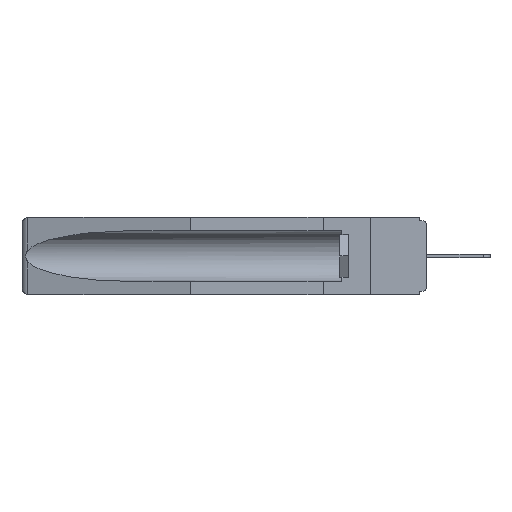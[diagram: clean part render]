
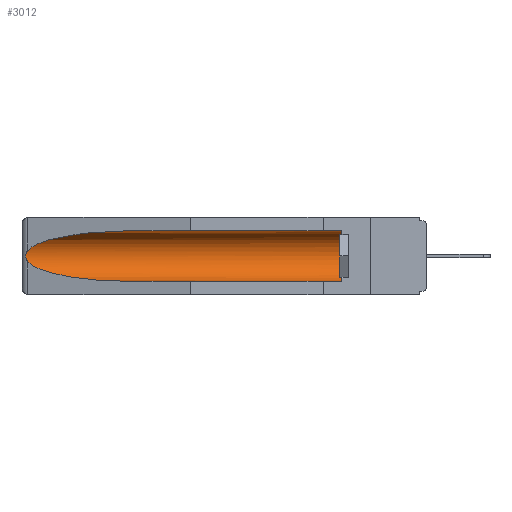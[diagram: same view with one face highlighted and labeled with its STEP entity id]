
A CAD part, left-side view. The second image highlights one B-rep face of the part: STEP entity #3012.
In plain terms, the highlighted cylindrical face has radius 2.857 mm (diameter 5.715 mm), a partial arc.
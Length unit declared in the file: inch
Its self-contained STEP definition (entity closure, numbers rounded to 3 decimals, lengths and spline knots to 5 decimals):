
#176 = CARTESIAN_POINT ( 'NONE',  ( 0.155, -0.30754, -0.284 ) ) ;
#478 = CARTESIAN_POINT ( 'NONE',  ( 0.2673, 1.5327, -0.16383 ) ) ;
#628 = CARTESIAN_POINT ( 'NONE',  ( 0.26654, 1.53092, -0.15636 ) ) ;
#876 = FACE_OUTER_BOUND ( 'NONE', #15188, .T. ) ;
#1124 = VERTEX_POINT ( 'NONE', #7832 ) ;
#1272 = CARTESIAN_POINT ( 'NONE',  ( 0.155, -0.30754, -0.1715 ) ) ;
#1479 =( BOUNDED_CURVE ( )  B_SPLINE_CURVE ( 3, ( #5331, #14253, #7152, #3442 ),
 .UNSPECIFIED., .F., .T. ) 
 B_SPLINE_CURVE_WITH_KNOTS ( ( 4, 4 ),
 ( 4.71239, 6.08839 ),
 .UNSPECIFIED. ) 
 CURVE ( )  GEOMETRIC_REPRESENTATION_ITEM ( )  RATIONAL_B_SPLINE_CURVE ( ( 1., 0.848, 0.848, 1. ) ) 
 REPRESENTATION_ITEM ( '' )  );
#1482 = VECTOR ( 'NONE', #19465, 39.37008 ) ;
#2046 = AXIS2_PLACEMENT_3D ( 'NONE', #1272, #12177, #14144 ) ;
#2461 = CARTESIAN_POINT ( 'NONE',  ( 0.26597, 1.5296, -0.19026 ) ) ;
#2616 = CARTESIAN_POINT ( 'NONE',  ( 0.155, 0.126, -0.059 ) ) ;
#3012 = ADVANCED_FACE ( 'NONE', ( #876 ), #17522, .F. ) ;
#3419 = DIRECTION ( 'NONE',  ( 0., 1., 0. ) ) ;
#3442 = CARTESIAN_POINT ( 'NONE',  ( 0.26537, 1.52718, -0.14972 ) ) ;
#3687 = LINE ( 'NONE', #176, #17489 ) ;
#4626 = B_SPLINE_CURVE_WITH_KNOTS ( 'NONE', 3,
 ( #7908, #22263, #628, #478, #9642, #9488, #7737, #11466, #2461, #16967 ),
 .UNSPECIFIED., .F., .F.,
 ( 4, 2, 2, 2, 4 ),
 ( 0., 0.00029, 0.00058, 0.00087, 0.00117 ),
 .UNSPECIFIED. ) ;
#5114 = EDGE_CURVE ( 'NONE', #10208, #1124, #1479, .T. ) ;
#5139 = CARTESIAN_POINT ( 'NONE',  ( 0.25451, 1.48313, -0.24835 ) ) ;
#5331 = CARTESIAN_POINT ( 'NONE',  ( 0.155, 1.07973, -0.059 ) ) ;
#5422 = LINE ( 'NONE', #17666, #1482 ) ;
#5429 = EDGE_CURVE ( 'NONE', #11168, #21065, #15094, .T. ) ;
#5938 = CIRCLE ( 'NONE', #5954, 0.1125 ) ;
#5954 = AXIS2_PLACEMENT_3D ( 'NONE', #11797, #15586, #22744 ) ;
#6505 = CARTESIAN_POINT ( 'NONE',  ( 0.26537, 1.52718, -0.19328 ) ) ;
#7048 = VERTEX_POINT ( 'NONE', #10441 ) ;
#7152 = CARTESIAN_POINT ( 'NONE',  ( 0.25451, 1.48313, -0.09465 ) ) ;
#7424 = CARTESIAN_POINT ( 'NONE',  ( 0.155, 1.07973, -0.284 ) ) ;
#7737 = CARTESIAN_POINT ( 'NONE',  ( 0.2673, 1.53269, -0.17917 ) ) ;
#7832 = CARTESIAN_POINT ( 'NONE',  ( 0.26537, 1.52718, -0.14972 ) ) ;
#7908 = CARTESIAN_POINT ( 'NONE',  ( 0.26537, 1.52718, -0.14972 ) ) ;
#9488 = CARTESIAN_POINT ( 'NONE',  ( 0.2675, 1.53308, -0.17534 ) ) ;
#9642 = CARTESIAN_POINT ( 'NONE',  ( 0.2675, 1.53308, -0.16763 ) ) ;
#9734 = EDGE_CURVE ( 'NONE', #7048, #12104, #5938, .T. ) ;
#10208 = VERTEX_POINT ( 'NONE', #18432 ) ;
#10441 = CARTESIAN_POINT ( 'NONE',  ( 0.155, 0.126, -0.284 ) ) ;
#10947 = ORIENTED_EDGE ( 'NONE', *, *, #9734, .T. ) ;
#11168 = VERTEX_POINT ( 'NONE', #6505 ) ;
#11466 = CARTESIAN_POINT ( 'NONE',  ( 0.26655, 1.53094, -0.18657 ) ) ;
#11646 = EDGE_CURVE ( 'NONE', #1124, #11168, #4626, .T. ) ;
#11797 = CARTESIAN_POINT ( 'NONE',  ( 0.155, 0.126, -0.1715 ) ) ;
#12104 = VERTEX_POINT ( 'NONE', #2616 ) ;
#12177 = DIRECTION ( 'NONE',  ( 0., 1., 0. ) ) ;
#14144 = DIRECTION ( 'NONE',  ( 0., 0., 1. ) ) ;
#14154 = CARTESIAN_POINT ( 'NONE',  ( 0.155, 1.07973, -0.284 ) ) ;
#14220 = CARTESIAN_POINT ( 'NONE',  ( 0.21114, 1.30732, -0.284 ) ) ;
#14253 = CARTESIAN_POINT ( 'NONE',  ( 0.21114, 1.30732, -0.059 ) ) ;
#14801 = ORIENTED_EDGE ( 'NONE', *, *, #5429, .T. ) ;
#15094 =( BOUNDED_CURVE ( )  B_SPLINE_CURVE ( 3, ( #15979, #5139, #14220, #7424 ),
 .UNSPECIFIED., .F., .T. ) 
 B_SPLINE_CURVE_WITH_KNOTS ( ( 4, 4 ),
 ( 0.1948, 1.5708 ),
 .UNSPECIFIED. ) 
 CURVE ( )  GEOMETRIC_REPRESENTATION_ITEM ( )  RATIONAL_B_SPLINE_CURVE ( ( 1., 0.848, 0.848, 1. ) ) 
 REPRESENTATION_ITEM ( '' )  );
#15188 = EDGE_LOOP ( 'NONE', ( #19473, #20785, #14801, #21242, #10947, #20935 ) ) ;
#15586 = DIRECTION ( 'NONE',  ( 0., -1., 0. ) ) ;
#15979 = CARTESIAN_POINT ( 'NONE',  ( 0.26537, 1.52718, -0.19328 ) ) ;
#16967 = CARTESIAN_POINT ( 'NONE',  ( 0.26537, 1.52718, -0.19328 ) ) ;
#17489 = VECTOR ( 'NONE', #3419, 39.37008 ) ;
#17522 = CYLINDRICAL_SURFACE ( 'NONE', #2046, 0.1125 ) ;
#17666 = CARTESIAN_POINT ( 'NONE',  ( 0.155, -0.30754, -0.059 ) ) ;
#18432 = CARTESIAN_POINT ( 'NONE',  ( 0.155, 1.07973, -0.059 ) ) ;
#18846 = EDGE_CURVE ( 'NONE', #7048, #21065, #3687, .T. ) ;
#19465 = DIRECTION ( 'NONE',  ( 0., 1., 0. ) ) ;
#19473 = ORIENTED_EDGE ( 'NONE', *, *, #5114, .T. ) ;
#20785 = ORIENTED_EDGE ( 'NONE', *, *, #11646, .T. ) ;
#20935 = ORIENTED_EDGE ( 'NONE', *, *, #23153, .T. ) ;
#21065 = VERTEX_POINT ( 'NONE', #14154 ) ;
#21242 = ORIENTED_EDGE ( 'NONE', *, *, #18846, .F. ) ;
#22263 = CARTESIAN_POINT ( 'NONE',  ( 0.26597, 1.52961, -0.15275 ) ) ;
#22744 = DIRECTION ( 'NONE',  ( 0., 0., 1. ) ) ;
#23153 = EDGE_CURVE ( 'NONE', #12104, #10208, #5422, .T. ) ;
